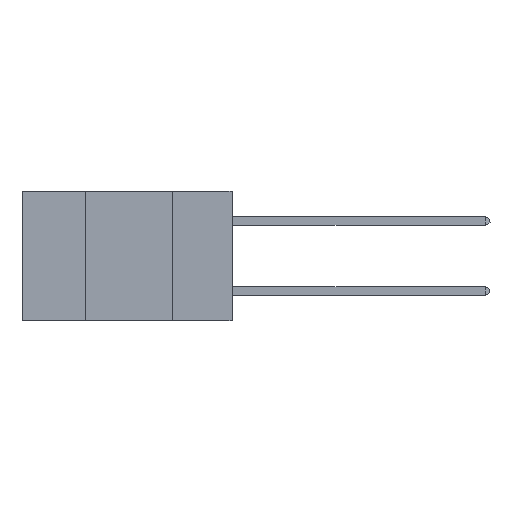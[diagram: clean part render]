
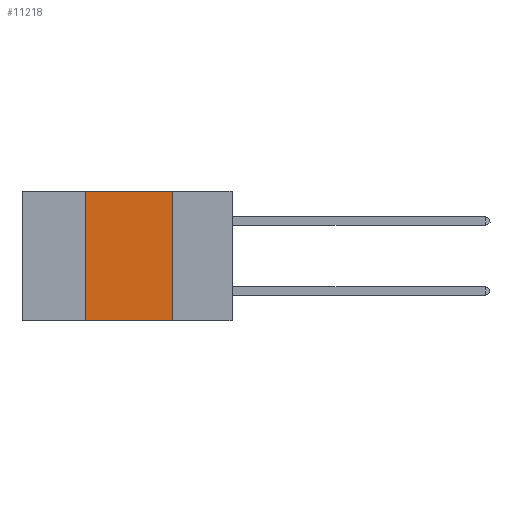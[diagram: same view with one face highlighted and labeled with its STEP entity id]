
A CAD part, left-side view. The second image highlights one B-rep face of the part: STEP entity #11218.
In plain terms, the highlighted planar face has unit normal (-1, 0, 0).
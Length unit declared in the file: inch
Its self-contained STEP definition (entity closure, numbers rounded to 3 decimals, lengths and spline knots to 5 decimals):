
#961 = CARTESIAN_POINT ( 'NONE',  ( 0., 0.6, 0. ) ) ;
#2443 = VECTOR ( 'NONE', #4893, 39.37008 ) ;
#2705 = EDGE_LOOP ( 'NONE', ( #12063, #14417, #9025, #5791 ) ) ;
#2866 = DIRECTION ( 'NONE',  ( 0., 0., -1. ) ) ;
#3000 = VERTEX_POINT ( 'NONE', #4833 ) ;
#3677 = CARTESIAN_POINT ( 'NONE',  ( 0., 0.42, 0. ) ) ;
#4064 = VERTEX_POINT ( 'NONE', #6255 ) ;
#4833 = CARTESIAN_POINT ( 'NONE',  ( 0., 0.42, 0. ) ) ;
#4893 = DIRECTION ( 'NONE',  ( 0., 0., 1. ) ) ;
#5236 = CARTESIAN_POINT ( 'NONE',  ( 0., 0.17, 0. ) ) ;
#5464 = LINE ( 'NONE', #14680, #11812 ) ;
#5791 = ORIENTED_EDGE ( 'NONE', *, *, #7640, .T. ) ;
#6255 = CARTESIAN_POINT ( 'NONE',  ( 0., 0.17, -0.37 ) ) ;
#6318 = LINE ( 'NONE', #961, #9851 ) ;
#6984 = EDGE_CURVE ( 'NONE', #3000, #9223, #6318, .T. ) ;
#7169 = EDGE_CURVE ( 'NONE', #9223, #4064, #5464, .T. ) ;
#7640 = EDGE_CURVE ( 'NONE', #8346, #4064, #12727, .T. ) ;
#7869 = CARTESIAN_POINT ( 'NONE',  ( 0., 0.42, -0.37 ) ) ;
#8346 = VERTEX_POINT ( 'NONE', #7869 ) ;
#9025 = ORIENTED_EDGE ( 'NONE', *, *, #16345, .F. ) ;
#9223 = VERTEX_POINT ( 'NONE', #5236 ) ;
#9671 = PLANE ( 'NONE',  #13684 ) ;
#9851 = VECTOR ( 'NONE', #14233, 39.37008 ) ;
#10872 = VECTOR ( 'NONE', #13999, 39.37008 ) ;
#11218 = ADVANCED_FACE ( 'NONE', ( #16995 ), #9671, .F. ) ;
#11812 = VECTOR ( 'NONE', #2866, 39.37008 ) ;
#12058 = DIRECTION ( 'NONE',  ( 1., 0., 0. ) ) ;
#12063 = ORIENTED_EDGE ( 'NONE', *, *, #7169, .F. ) ;
#12727 = LINE ( 'NONE', #13763, #10872 ) ;
#13346 = CARTESIAN_POINT ( 'NONE',  ( 0., 0.6, 0. ) ) ;
#13684 = AXIS2_PLACEMENT_3D ( 'NONE', #13346, #12058, #14546 ) ;
#13763 = CARTESIAN_POINT ( 'NONE',  ( 0., 0.6, -0.37 ) ) ;
#13999 = DIRECTION ( 'NONE',  ( 0., -1., 0. ) ) ;
#14233 = DIRECTION ( 'NONE',  ( 0., -1., 0. ) ) ;
#14417 = ORIENTED_EDGE ( 'NONE', *, *, #6984, .F. ) ;
#14546 = DIRECTION ( 'NONE',  ( 0., 0., -1. ) ) ;
#14680 = CARTESIAN_POINT ( 'NONE',  ( 0., 0.17, 0. ) ) ;
#15330 = LINE ( 'NONE', #3677, #2443 ) ;
#16345 = EDGE_CURVE ( 'NONE', #8346, #3000, #15330, .T. ) ;
#16995 = FACE_OUTER_BOUND ( 'NONE', #2705, .T. ) ;
